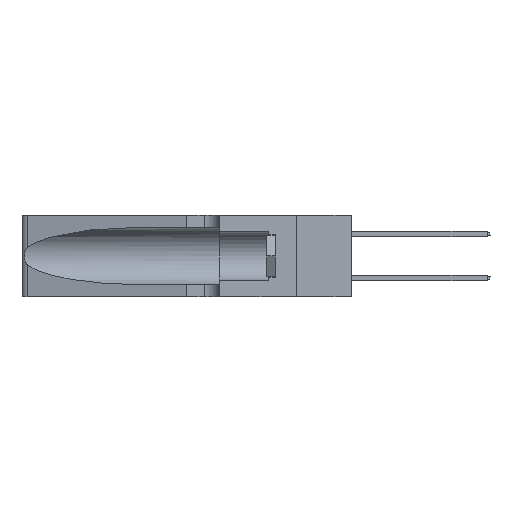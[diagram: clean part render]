
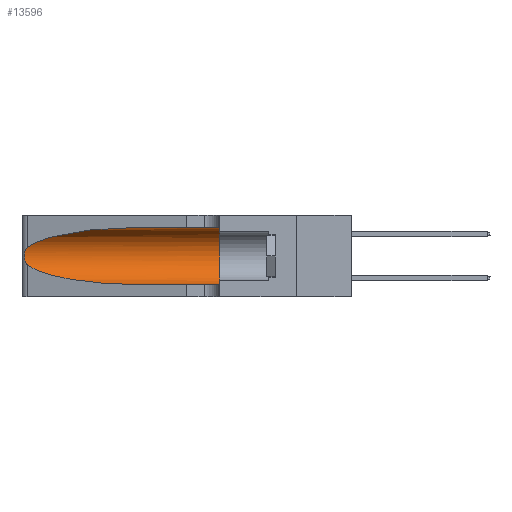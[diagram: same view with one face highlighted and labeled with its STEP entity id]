
A CAD part, left-side view. The second image highlights one B-rep face of the part: STEP entity #13596.
In plain terms, the highlighted cylindrical face has radius 3.308 mm (diameter 6.617 mm), a partial arc.
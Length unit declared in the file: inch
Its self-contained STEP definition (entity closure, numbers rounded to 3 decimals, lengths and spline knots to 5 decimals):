
#957 = VECTOR ( 'NONE', #24246, 39.37008 ) ;
#972 = CIRCLE ( 'NONE', #33324, 0.13025 ) ;
#1240 = CARTESIAN_POINT ( 'NONE',  ( 0.25487, 1.22718, 0.14631 ) ) ;
#1836 = CARTESIAN_POINT ( 'NONE',  ( 0.25487, 1.22718, 0.22369 ) ) ;
#2296 = CARTESIAN_POINT ( 'NONE',  ( 0.25639, 1.23186, 0.15144 ) ) ;
#2663 = EDGE_CURVE ( 'NONE', #7116, #30155, #10248, .T. ) ;
#2814 = CARTESIAN_POINT ( 'NONE',  ( 0.25487, 1.22718, 0.14631 ) ) ;
#2838 = CARTESIAN_POINT ( 'NONE',  ( 0.25487, 1.22718, 0.14631 ) ) ;
#3323 = VERTEX_POINT ( 'NONE', #27680 ) ;
#3769 = ORIENTED_EDGE ( 'NONE', *, *, #5495, .T. ) ;
#5495 = EDGE_CURVE ( 'NONE', #30909, #25653, #15047, .T. ) ;
#7116 = VERTEX_POINT ( 'NONE', #12694 ) ;
#8057 = ORIENTED_EDGE ( 'NONE', *, *, #30789, .T. ) ;
#8382 = CARTESIAN_POINT ( 'NONE',  ( 0.25787, 1.23484, 0.2124 ) ) ;
#8467 = CARTESIAN_POINT ( 'NONE',  ( 0.26075, 1.23896, 0.19203 ) ) ;
#8513 = FACE_OUTER_BOUND ( 'NONE', #28447, .T. ) ;
#9605 = CARTESIAN_POINT ( 'NONE',  ( 0.1305, 0.72297, 0.31525 ) ) ;
#10248 = LINE ( 'NONE', #36303, #957 ) ;
#11773 = CARTESIAN_POINT ( 'NONE',  ( 0.2373, 1.15595, 0.08982 ) ) ;
#12694 = CARTESIAN_POINT ( 'NONE',  ( 0.1305, 0.72297, 0.05475 ) ) ;
#13251 = CARTESIAN_POINT ( 'NONE',  ( 0.18966, 0.96281, 0.31525 ) ) ;
#13256 = CARTESIAN_POINT ( 'NONE',  ( 0.25639, 1.23184, 0.21858 ) ) ;
#13596 = ADVANCED_FACE ( 'NONE', ( #8513 ), #25663, .F. ) ;
#14345 = CARTESIAN_POINT ( 'NONE',  ( 0.26018, 1.23835, 0.19895 ) ) ;
#14597 = CARTESIAN_POINT ( 'NONE',  ( 0.1305, 1.61858, 0.31525 ) ) ;
#14614 = CARTESIAN_POINT ( 'NONE',  ( 0.26017, 1.23833, 0.17102 ) ) ;
#14645 = CARTESIAN_POINT ( 'NONE',  ( 0.18966, 0.96281, 0.05475 ) ) ;
#15047 = B_SPLINE_CURVE_WITH_KNOTS ( 'NONE', 3,
 ( #22213, #30987, #13256, #8382, #29341, #14345, #8467, #17466, #14614, #34963, #32230, #2296, #35105, #2814 ),
 .UNSPECIFIED., .F., .F.,
 ( 4, 2, 2, 2, 2, 2, 4 ),
 ( 0., 0.00027, 0.00053, 0.00107, 0.0016, 0.00187, 0.00214 ),
 .UNSPECIFIED. ) ;
#15151 = DIRECTION ( 'NONE',  ( 0., 0., 1. ) ) ;
#17466 = CARTESIAN_POINT ( 'NONE',  ( 0.26075, 1.23896, 0.178 ) ) ;
#18343 = EDGE_CURVE ( 'NONE', #29872, #30909, #22388, .T. ) ;
#18677 = ORIENTED_EDGE ( 'NONE', *, *, #26033, .F. ) ;
#21330 = CARTESIAN_POINT ( 'NONE',  ( 0.25487, 1.22718, 0.22369 ) ) ;
#22213 = CARTESIAN_POINT ( 'NONE',  ( 0.25487, 1.22718, 0.22369 ) ) ;
#22388 =( BOUNDED_CURVE ( )  B_SPLINE_CURVE ( 3, ( #9605, #13251, #37088, #1836 ),
 .UNSPECIFIED., .F., .T. ) 
 B_SPLINE_CURVE_WITH_KNOTS ( ( 4, 4 ),
 ( 1.5708, 2.84003 ),
 .UNSPECIFIED. ) 
 CURVE ( )  GEOMETRIC_REPRESENTATION_ITEM ( )  RATIONAL_B_SPLINE_CURVE ( ( 1., 0.87, 0.87, 1. ) ) 
 REPRESENTATION_ITEM ( '' )  );
#23091 = DIRECTION ( 'NONE',  ( 0., -1., 0. ) ) ;
#23729 = ORIENTED_EDGE ( 'NONE', *, *, #27773, .F. ) ;
#24034 = VECTOR ( 'NONE', #26623, 39.37008 ) ;
#24246 = DIRECTION ( 'NONE',  ( 0., -1., 0. ) ) ;
#25653 = VERTEX_POINT ( 'NONE', #1240 ) ;
#25663 = CYLINDRICAL_SURFACE ( 'NONE', #38388, 0.13025 ) ;
#25929 =( BOUNDED_CURVE ( )  B_SPLINE_CURVE ( 3, ( #2838, #11773, #14645, #32513 ),
 .UNSPECIFIED., .F., .F. ) 
 B_SPLINE_CURVE_WITH_KNOTS ( ( 4, 4 ),
 ( 3.44316, 4.71239 ),
 .UNSPECIFIED. ) 
 CURVE ( )  GEOMETRIC_REPRESENTATION_ITEM ( )  RATIONAL_B_SPLINE_CURVE ( ( 1., 0.87, 0.87, 1. ) ) 
 REPRESENTATION_ITEM ( '' )  );
#26033 = EDGE_CURVE ( 'NONE', #3323, #30155, #972, .T. ) ;
#26137 = CARTESIAN_POINT ( 'NONE',  ( 0.1305, 0.35, 0.185 ) ) ;
#26623 = DIRECTION ( 'NONE',  ( 0., -1., 0. ) ) ;
#27680 = CARTESIAN_POINT ( 'NONE',  ( 0.1305, 0.35, 0.31525 ) ) ;
#27773 = EDGE_CURVE ( 'NONE', #29872, #3323, #35673, .T. ) ;
#28447 = EDGE_LOOP ( 'NONE', ( #32233, #3769, #8057, #38146, #18677, #23729 ) ) ;
#29341 = CARTESIAN_POINT ( 'NONE',  ( 0.25854, 1.2359, 0.20912 ) ) ;
#29491 = DIRECTION ( 'NONE',  ( 0., 1., 0. ) ) ;
#29872 = VERTEX_POINT ( 'NONE', #36920 ) ;
#30155 = VERTEX_POINT ( 'NONE', #32536 ) ;
#30789 = EDGE_CURVE ( 'NONE', #25653, #7116, #25929, .T. ) ;
#30909 = VERTEX_POINT ( 'NONE', #21330 ) ;
#30987 = CARTESIAN_POINT ( 'NONE',  ( 0.25555, 1.22994, 0.2215 ) ) ;
#32171 = CARTESIAN_POINT ( 'NONE',  ( 0.1305, 1.61858, 0.185 ) ) ;
#32230 = CARTESIAN_POINT ( 'NONE',  ( 0.25789, 1.23486, 0.15765 ) ) ;
#32233 = ORIENTED_EDGE ( 'NONE', *, *, #18343, .T. ) ;
#32427 = DIRECTION ( 'NONE',  ( 0., 0., -1. ) ) ;
#32513 = CARTESIAN_POINT ( 'NONE',  ( 0.1305, 0.72297, 0.05475 ) ) ;
#32536 = CARTESIAN_POINT ( 'NONE',  ( 0.1305, 0.35, 0.05475 ) ) ;
#33324 = AXIS2_PLACEMENT_3D ( 'NONE', #26137, #29491, #15151 ) ;
#34963 = CARTESIAN_POINT ( 'NONE',  ( 0.25856, 1.23593, 0.16098 ) ) ;
#35105 = CARTESIAN_POINT ( 'NONE',  ( 0.25555, 1.22993, 0.14849 ) ) ;
#35673 = LINE ( 'NONE', #14597, #24034 ) ;
#36303 = CARTESIAN_POINT ( 'NONE',  ( 0.1305, 1.61858, 0.05475 ) ) ;
#36920 = CARTESIAN_POINT ( 'NONE',  ( 0.1305, 0.72297, 0.31525 ) ) ;
#37088 = CARTESIAN_POINT ( 'NONE',  ( 0.2373, 1.15595, 0.28018 ) ) ;
#38146 = ORIENTED_EDGE ( 'NONE', *, *, #2663, .T. ) ;
#38388 = AXIS2_PLACEMENT_3D ( 'NONE', #32171, #23091, #32427 ) ;
